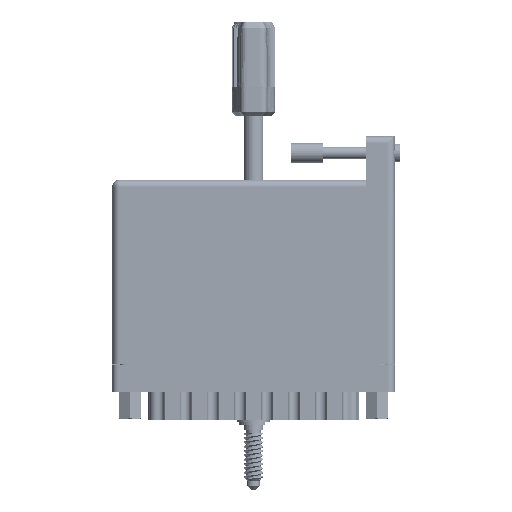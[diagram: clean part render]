
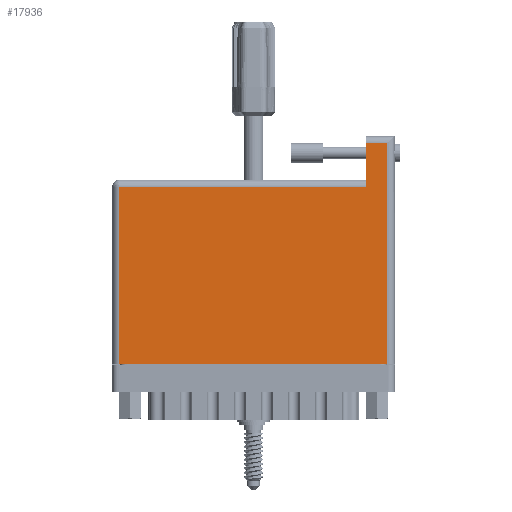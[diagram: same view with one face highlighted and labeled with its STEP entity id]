
A CAD part, front view. The second image highlights one B-rep face of the part: STEP entity #17936.
In plain terms, the highlighted face is planar.
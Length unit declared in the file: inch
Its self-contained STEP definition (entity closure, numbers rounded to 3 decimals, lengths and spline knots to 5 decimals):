
#454 = EDGE_LOOP ( 'NONE', ( #8525, #67975, #96461, #96254, #8205, #36409 ) ) ;
#3356 = VECTOR ( 'NONE', #26650, 39.37008 ) ;
#3942 = VECTOR ( 'NONE', #71623, 39.37008 ) ;
#4755 = LINE ( 'NONE', #28381, #77712 ) ;
#5225 = LINE ( 'NONE', #25907, #11152 ) ;
#8205 = ORIENTED_EDGE ( 'NONE', *, *, #78371, .T. ) ;
#8525 = ORIENTED_EDGE ( 'NONE', *, *, #90193, .T. ) ;
#9850 = CARTESIAN_POINT ( 'NONE',  ( 0., 0., 0. ) ) ;
#11152 = VECTOR ( 'NONE', #71219, 39.37008 ) ;
#13707 = DIRECTION ( 'NONE',  ( -1., 0., 0. ) ) ;
#14339 = CARTESIAN_POINT ( 'NONE',  ( 0., 2.125, 0. ) ) ;
#17936 = ADVANCED_FACE ( 'NONE', ( #71158 ), #50309, .F. ) ;
#18311 = CARTESIAN_POINT ( 'NONE',  ( 2.438, 2.195, 0. ) ) ;
#19995 = DIRECTION ( 'NONE',  ( 0., 0., -1. ) ) ;
#22338 = VECTOR ( 'NONE', #48114, 39.37008 ) ;
#22523 = CARTESIAN_POINT ( 'NONE',  ( 2.438, 2.125, 0. ) ) ;
#25907 = CARTESIAN_POINT ( 'NONE',  ( 0.07, 0., 0. ) ) ;
#25914 = CARTESIAN_POINT ( 'NONE',  ( 2.648, 2.125, 0. ) ) ;
#26422 = CARTESIAN_POINT ( 'NONE',  ( 2.648, 0., 0. ) ) ;
#26650 = DIRECTION ( 'NONE',  ( -1., 0., 0. ) ) ;
#28381 = CARTESIAN_POINT ( 'NONE',  ( 2.648, 2.195, 0. ) ) ;
#33175 = VERTEX_POINT ( 'NONE', #34412 ) ;
#34412 = CARTESIAN_POINT ( 'NONE',  ( 0.07, 0., 0. ) ) ;
#36409 = ORIENTED_EDGE ( 'NONE', *, *, #87448, .T. ) ;
#37429 = EDGE_CURVE ( 'NONE', #33175, #96782, #40179, .T. ) ;
#40179 = LINE ( 'NONE', #9850, #22338 ) ;
#41929 = EDGE_CURVE ( 'NONE', #96782, #64559, #4755, .T. ) ;
#41998 = DIRECTION ( 'NONE',  ( -1., 0., 0. ) ) ;
#42920 = CARTESIAN_POINT ( 'NONE',  ( 0., 1.705, 0. ) ) ;
#48114 = DIRECTION ( 'NONE',  ( 1., 0., 0. ) ) ;
#50309 = PLANE ( 'NONE',  #89656 ) ;
#54653 = LINE ( 'NONE', #42920, #3356 ) ;
#55945 = EDGE_CURVE ( 'NONE', #96602, #33175, #5225, .T. ) ;
#64559 = VERTEX_POINT ( 'NONE', #25914 ) ;
#67975 = ORIENTED_EDGE ( 'NONE', *, *, #55945, .T. ) ;
#71158 = FACE_OUTER_BOUND ( 'NONE', #454, .T. ) ;
#71219 = DIRECTION ( 'NONE',  ( 0., -1., 0. ) ) ;
#71623 = DIRECTION ( 'NONE',  ( 0., -1., 0. ) ) ;
#75960 = CARTESIAN_POINT ( 'NONE',  ( 2.438, 1.705, 0. ) ) ;
#77712 = VECTOR ( 'NONE', #89955, 39.37008 ) ;
#78371 = EDGE_CURVE ( 'NONE', #64559, #91966, #92372, .T. ) ;
#86116 = LINE ( 'NONE', #18311, #3942 ) ;
#87448 = EDGE_CURVE ( 'NONE', #91966, #97720, #86116, .T. ) ;
#87623 = CARTESIAN_POINT ( 'NONE',  ( 0., 1.775, 0. ) ) ;
#89656 = AXIS2_PLACEMENT_3D ( 'NONE', #87623, #19995, #41998 ) ;
#89955 = DIRECTION ( 'NONE',  ( 0., 1., 0. ) ) ;
#90193 = EDGE_CURVE ( 'NONE', #97720, #96602, #54653, .T. ) ;
#90388 = CARTESIAN_POINT ( 'NONE',  ( 0.07, 1.705, 0. ) ) ;
#91966 = VERTEX_POINT ( 'NONE', #22523 ) ;
#92372 = LINE ( 'NONE', #14339, #95932 ) ;
#95932 = VECTOR ( 'NONE', #13707, 39.37008 ) ;
#96254 = ORIENTED_EDGE ( 'NONE', *, *, #41929, .T. ) ;
#96461 = ORIENTED_EDGE ( 'NONE', *, *, #37429, .T. ) ;
#96602 = VERTEX_POINT ( 'NONE', #90388 ) ;
#96782 = VERTEX_POINT ( 'NONE', #26422 ) ;
#97720 = VERTEX_POINT ( 'NONE', #75960 ) ;
